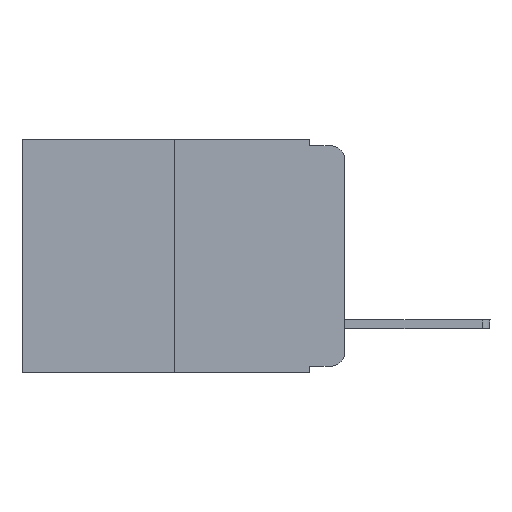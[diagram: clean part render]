
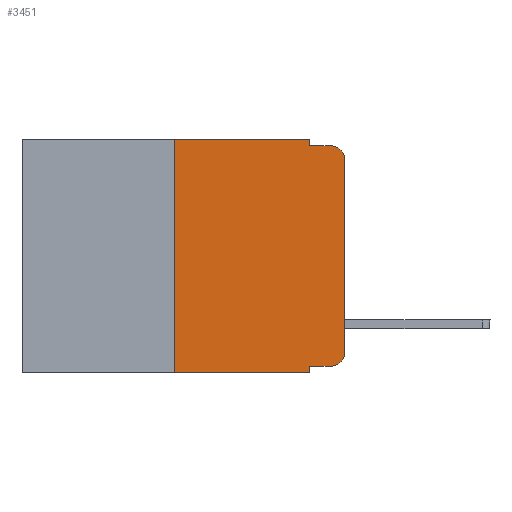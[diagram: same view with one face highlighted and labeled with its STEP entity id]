
A CAD part, left-side view. The second image highlights one B-rep face of the part: STEP entity #3451.
In plain terms, the highlighted planar face has unit normal (-1, 0, 0).
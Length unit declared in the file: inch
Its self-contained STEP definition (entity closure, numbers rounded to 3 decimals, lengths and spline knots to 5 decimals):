
#334 = CARTESIAN_POINT ( 'NONE',  ( 0., 0.051, -0.333 ) ) ;
#512 = CARTESIAN_POINT ( 'NONE',  ( 0., 0.051, -0.343 ) ) ;
#800 = CARTESIAN_POINT ( 'NONE',  ( 0., 0.051, -0.01 ) ) ;
#838 = DIRECTION ( 'NONE',  ( 0., -1., 0. ) ) ;
#927 = LINE ( 'NONE', #4074, #5971 ) ;
#1028 = ORIENTED_EDGE ( 'NONE', *, *, #12375, .F. ) ;
#1181 = CARTESIAN_POINT ( 'NONE',  ( 0., 0.051, -0.01 ) ) ;
#1447 = LINE ( 'NONE', #1181, #1773 ) ;
#1755 = EDGE_LOOP ( 'NONE', ( #13279, #8754, #6116, #1028, #4641, #2502, #3754, #3940, #6219, #7504 ) ) ;
#1773 = VECTOR ( 'NONE', #6527, 39.37008 ) ;
#2104 = CARTESIAN_POINT ( 'NONE',  ( 0., 0.02, -0.313 ) ) ;
#2178 = VERTEX_POINT ( 'NONE', #7499 ) ;
#2359 = AXIS2_PLACEMENT_3D ( 'NONE', #2104, #10886, #10749 ) ;
#2502 = ORIENTED_EDGE ( 'NONE', *, *, #10472, .F. ) ;
#2545 = DIRECTION ( 'NONE',  ( 0., 0., -1. ) ) ;
#2648 = VECTOR ( 'NONE', #9443, 39.37008 ) ;
#3280 = FACE_OUTER_BOUND ( 'NONE', #1755, .T. ) ;
#3345 = DIRECTION ( 'NONE',  ( -1., 0., 0. ) ) ;
#3383 = DIRECTION ( 'NONE',  ( 0., 0., 1. ) ) ;
#3451 = ADVANCED_FACE ( 'NONE', ( #3280 ), #3713, .F. ) ;
#3506 = CARTESIAN_POINT ( 'NONE',  ( 0., 0.02, -0.01 ) ) ;
#3600 = CARTESIAN_POINT ( 'NONE',  ( 0., 0.473, 0. ) ) ;
#3604 = LINE ( 'NONE', #12647, #4618 ) ;
#3713 = PLANE ( 'NONE',  #10577 ) ;
#3751 = EDGE_CURVE ( 'NONE', #6362, #2178, #3604, .T. ) ;
#3754 = ORIENTED_EDGE ( 'NONE', *, *, #8712, .T. ) ;
#3788 = EDGE_CURVE ( 'NONE', #5645, #13216, #1447, .T. ) ;
#3940 = ORIENTED_EDGE ( 'NONE', *, *, #8898, .F. ) ;
#4053 = EDGE_CURVE ( 'NONE', #10694, #5664, #9343, .T. ) ;
#4074 = CARTESIAN_POINT ( 'NONE',  ( 0., 0.25, 0. ) ) ;
#4444 = DIRECTION ( 'NONE',  ( 0., 0., -1. ) ) ;
#4462 = CARTESIAN_POINT ( 'NONE',  ( 0., 0.051, 0. ) ) ;
#4618 = VECTOR ( 'NONE', #838, 39.37008 ) ;
#4641 = ORIENTED_EDGE ( 'NONE', *, *, #4053, .F. ) ;
#5028 = CARTESIAN_POINT ( 'NONE',  ( 0., 0., -0.313 ) ) ;
#5193 = CARTESIAN_POINT ( 'NONE',  ( 0., 0.051, 0. ) ) ;
#5525 = VECTOR ( 'NONE', #13716, 39.37008 ) ;
#5616 = CARTESIAN_POINT ( 'NONE',  ( 0., 0.02, -0.03 ) ) ;
#5645 = VERTEX_POINT ( 'NONE', #800 ) ;
#5664 = VERTEX_POINT ( 'NONE', #12780 ) ;
#5811 = VECTOR ( 'NONE', #13287, 39.37008 ) ;
#5904 = CARTESIAN_POINT ( 'NONE',  ( 0., 0.25, 0. ) ) ;
#5971 = VECTOR ( 'NONE', #10575, 39.37008 ) ;
#6116 = ORIENTED_EDGE ( 'NONE', *, *, #3788, .F. ) ;
#6219 = ORIENTED_EDGE ( 'NONE', *, *, #3751, .T. ) ;
#6362 = VERTEX_POINT ( 'NONE', #334 ) ;
#6527 = DIRECTION ( 'NONE',  ( 0., -1., 0. ) ) ;
#6780 = LINE ( 'NONE', #5193, #10665 ) ;
#7148 = CARTESIAN_POINT ( 'NONE',  ( 0., 0.473, -0.343 ) ) ;
#7392 = VERTEX_POINT ( 'NONE', #512 ) ;
#7466 = LINE ( 'NONE', #12937, #8816 ) ;
#7499 = CARTESIAN_POINT ( 'NONE',  ( 0., 0.02, -0.333 ) ) ;
#7504 = ORIENTED_EDGE ( 'NONE', *, *, #11169, .T. ) ;
#7592 = VERTEX_POINT ( 'NONE', #11785 ) ;
#7723 = EDGE_CURVE ( 'NONE', #13733, #13216, #9905, .T. ) ;
#8712 = EDGE_CURVE ( 'NONE', #7592, #7392, #8889, .T. ) ;
#8754 = ORIENTED_EDGE ( 'NONE', *, *, #7723, .T. ) ;
#8816 = VECTOR ( 'NONE', #3383, 39.37008 ) ;
#8889 = LINE ( 'NONE', #7148, #5525 ) ;
#8898 = EDGE_CURVE ( 'NONE', #6362, #7392, #13083, .T. ) ;
#8899 = DIRECTION ( 'NONE',  ( 1., 0., 0. ) ) ;
#9343 = LINE ( 'NONE', #3600, #5811 ) ;
#9443 = DIRECTION ( 'NONE',  ( 0., 0., -1. ) ) ;
#9648 = CARTESIAN_POINT ( 'NONE',  ( 0., 0., -0.03 ) ) ;
#9905 = CIRCLE ( 'NONE', #10151, 0.02 ) ;
#10151 = AXIS2_PLACEMENT_3D ( 'NONE', #5616, #3345, #4444 ) ;
#10301 = VERTEX_POINT ( 'NONE', #5028 ) ;
#10472 = EDGE_CURVE ( 'NONE', #7592, #10694, #927, .T. ) ;
#10531 = CARTESIAN_POINT ( 'NONE',  ( 0., 0.473, 0. ) ) ;
#10575 = DIRECTION ( 'NONE',  ( 0., 0., 1. ) ) ;
#10577 = AXIS2_PLACEMENT_3D ( 'NONE', #10531, #8899, #2545 ) ;
#10665 = VECTOR ( 'NONE', #13692, 39.37008 ) ;
#10694 = VERTEX_POINT ( 'NONE', #5904 ) ;
#10749 = DIRECTION ( 'NONE',  ( 0., 0., -1. ) ) ;
#10886 = DIRECTION ( 'NONE',  ( -1., 0., 0. ) ) ;
#11169 = EDGE_CURVE ( 'NONE', #2178, #10301, #12023, .T. ) ;
#11785 = CARTESIAN_POINT ( 'NONE',  ( 0., 0.25, -0.343 ) ) ;
#12023 = CIRCLE ( 'NONE', #2359, 0.02 ) ;
#12375 = EDGE_CURVE ( 'NONE', #5664, #5645, #6780, .T. ) ;
#12647 = CARTESIAN_POINT ( 'NONE',  ( 0., 0.051, -0.333 ) ) ;
#12780 = CARTESIAN_POINT ( 'NONE',  ( 0., 0.051, 0. ) ) ;
#12937 = CARTESIAN_POINT ( 'NONE',  ( 0., 0., 0. ) ) ;
#13083 = LINE ( 'NONE', #4462, #2648 ) ;
#13216 = VERTEX_POINT ( 'NONE', #3506 ) ;
#13279 = ORIENTED_EDGE ( 'NONE', *, *, #13893, .T. ) ;
#13287 = DIRECTION ( 'NONE',  ( 0., -1., 0. ) ) ;
#13692 = DIRECTION ( 'NONE',  ( 0., 0., -1. ) ) ;
#13716 = DIRECTION ( 'NONE',  ( 0., -1., 0. ) ) ;
#13733 = VERTEX_POINT ( 'NONE', #9648 ) ;
#13893 = EDGE_CURVE ( 'NONE', #10301, #13733, #7466, .T. ) ;
